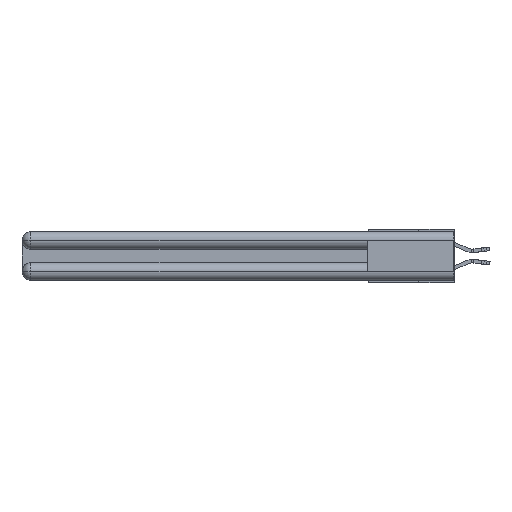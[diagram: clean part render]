
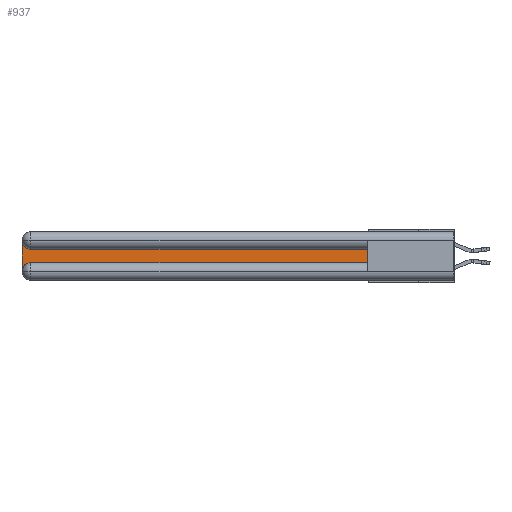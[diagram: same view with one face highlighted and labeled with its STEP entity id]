
A CAD part, left-side view. The second image highlights one B-rep face of the part: STEP entity #937.
In plain terms, the highlighted planar face has unit normal (-1, 0, 0).
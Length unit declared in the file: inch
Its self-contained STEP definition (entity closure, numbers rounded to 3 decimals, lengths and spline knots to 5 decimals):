
#4 = CARTESIAN_POINT ( 'NONE',  ( 0.075, 2.94, -0.1225 ) ) ;
#25 = DIRECTION ( 'NONE',  ( 0., 0., -1. ) ) ;
#559 = ORIENTED_EDGE ( 'NONE', *, *, #11321, .T. ) ;
#937 = ADVANCED_FACE ( 'NONE', ( #16305 ), #9985, .F. ) ;
#2379 = CIRCLE ( 'NONE', #25245, 0.06 ) ;
#2559 = DIRECTION ( 'NONE',  ( 0., 0., -1. ) ) ;
#2733 = LINE ( 'NONE', #22019, #13816 ) ;
#5260 = VECTOR ( 'NONE', #12853, 39.37008 ) ;
#6104 = EDGE_CURVE ( 'NONE', #24981, #29214, #29783, .T. ) ;
#7821 = LINE ( 'NONE', #19477, #5260 ) ;
#8114 = DIRECTION ( 'NONE',  ( 0., 0., 1. ) ) ;
#8534 = CARTESIAN_POINT ( 'NONE',  ( 0.075, 0.6, -0.1225 ) ) ;
#9985 = PLANE ( 'NONE',  #19924 ) ;
#11321 = EDGE_CURVE ( 'NONE', #27742, #24981, #2733, .T. ) ;
#12853 = DIRECTION ( 'NONE',  ( 0., 0., -1. ) ) ;
#13179 = DIRECTION ( 'NONE',  ( 1., 0., 0. ) ) ;
#13613 = ORIENTED_EDGE ( 'NONE', *, *, #6104, .T. ) ;
#13629 = CIRCLE ( 'NONE', #21891, 0.06 ) ;
#13816 = VECTOR ( 'NONE', #8114, 39.37008 ) ;
#15581 = CARTESIAN_POINT ( 'NONE',  ( 0.075, 2.94, -0.2175 ) ) ;
#16305 = FACE_OUTER_BOUND ( 'NONE', #29242, .T. ) ;
#16424 = VECTOR ( 'NONE', #22990, 39.37008 ) ;
#17653 = CARTESIAN_POINT ( 'NONE',  ( 0.075, 3., -0.2775 ) ) ;
#17889 = DIRECTION ( 'NONE',  ( 1., 0., 0. ) ) ;
#18981 = ORIENTED_EDGE ( 'NONE', *, *, #25467, .T. ) ;
#19288 = ORIENTED_EDGE ( 'NONE', *, *, #35365, .T. ) ;
#19477 = CARTESIAN_POINT ( 'NONE',  ( 0.075, 3., -0.2175 ) ) ;
#19924 = AXIS2_PLACEMENT_3D ( 'NONE', #32348, #27385, #25 ) ;
#20601 = EDGE_CURVE ( 'NONE', #26796, #27742, #30570, .T. ) ;
#20873 = ORIENTED_EDGE ( 'NONE', *, *, #20601, .T. ) ;
#21891 = AXIS2_PLACEMENT_3D ( 'NONE', #29410, #13179, #2559 ) ;
#21990 = DIRECTION ( 'NONE',  ( 0., -1., 0. ) ) ;
#22019 = CARTESIAN_POINT ( 'NONE',  ( 0.075, 0.6, -0.2175 ) ) ;
#22990 = DIRECTION ( 'NONE',  ( 0., 1., 0. ) ) ;
#24298 = ORIENTED_EDGE ( 'NONE', *, *, #32529, .T. ) ;
#24981 = VERTEX_POINT ( 'NONE', #8534 ) ;
#25245 = AXIS2_PLACEMENT_3D ( 'NONE', #31356, #17889, #31578 ) ;
#25467 = EDGE_CURVE ( 'NONE', #29214, #32853, #2379, .T. ) ;
#25526 = VERTEX_POINT ( 'NONE', #17653 ) ;
#26211 = CARTESIAN_POINT ( 'NONE',  ( 0.075, 0.6, -0.2175 ) ) ;
#26796 = VERTEX_POINT ( 'NONE', #15581 ) ;
#27385 = DIRECTION ( 'NONE',  ( 1., 0., 0. ) ) ;
#27742 = VERTEX_POINT ( 'NONE', #26211 ) ;
#29214 = VERTEX_POINT ( 'NONE', #4 ) ;
#29242 = EDGE_LOOP ( 'NONE', ( #13613, #18981, #19288, #24298, #20873, #559 ) ) ;
#29410 = CARTESIAN_POINT ( 'NONE',  ( 0.075, 2.94, -0.2775 ) ) ;
#29783 = LINE ( 'NONE', #34111, #16424 ) ;
#30570 = LINE ( 'NONE', #30808, #33611 ) ;
#30808 = CARTESIAN_POINT ( 'NONE',  ( 0.075, 0.6, -0.2175 ) ) ;
#30924 = CARTESIAN_POINT ( 'NONE',  ( 0.075, 3., -0.0625 ) ) ;
#31356 = CARTESIAN_POINT ( 'NONE',  ( 0.075, 2.94, -0.0625 ) ) ;
#31578 = DIRECTION ( 'NONE',  ( 0., 0., -1. ) ) ;
#32348 = CARTESIAN_POINT ( 'NONE',  ( 0.075, 3., -0.1225 ) ) ;
#32529 = EDGE_CURVE ( 'NONE', #25526, #26796, #13629, .T. ) ;
#32853 = VERTEX_POINT ( 'NONE', #30924 ) ;
#33611 = VECTOR ( 'NONE', #21990, 39.37008 ) ;
#34111 = CARTESIAN_POINT ( 'NONE',  ( 0.075, 0.6, -0.1225 ) ) ;
#35365 = EDGE_CURVE ( 'NONE', #32853, #25526, #7821, .T. ) ;
